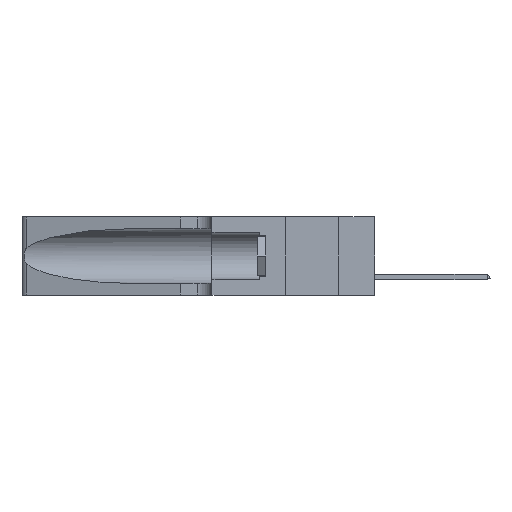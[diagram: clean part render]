
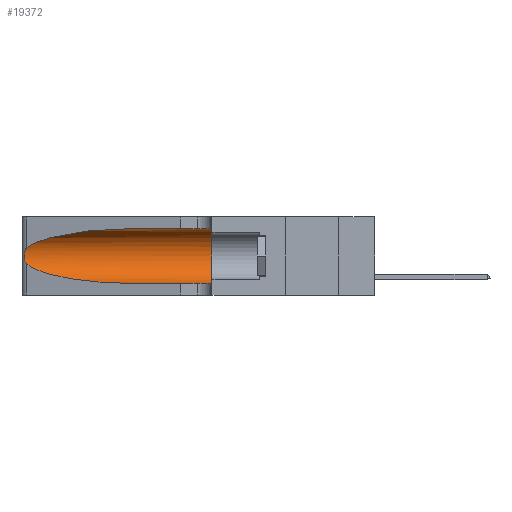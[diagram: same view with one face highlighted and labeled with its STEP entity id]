
A CAD part, left-side view. The second image highlights one B-rep face of the part: STEP entity #19372.
In plain terms, the highlighted cylindrical face has radius 3.308 mm (diameter 6.617 mm), a partial arc.
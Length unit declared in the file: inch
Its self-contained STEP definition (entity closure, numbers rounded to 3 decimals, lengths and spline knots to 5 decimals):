
#182 = DIRECTION ( 'NONE',  ( 0., -1., 0. ) ) ;
#310 = CARTESIAN_POINT ( 'NONE',  ( 0.18966, 0.96281, 0.31525 ) ) ;
#332 = DIRECTION ( 'NONE',  ( 0., -1., 0. ) ) ;
#604 = ORIENTED_EDGE ( 'NONE', *, *, #14429, .T. ) ;
#1430 = CIRCLE ( 'NONE', #5214, 0.13025 ) ;
#1632 = FACE_OUTER_BOUND ( 'NONE', #19201, .T. ) ;
#1670 = CARTESIAN_POINT ( 'NONE',  ( 0.1305, 0.72297, 0.05475 ) ) ;
#1849 = CARTESIAN_POINT ( 'NONE',  ( 0.1305, 1.61858, 0.05475 ) ) ;
#1985 = CARTESIAN_POINT ( 'NONE',  ( 0.1305, 0.35, 0.05475 ) ) ;
#2293 = CARTESIAN_POINT ( 'NONE',  ( 0.25854, 1.2359, 0.20912 ) ) ;
#2386 = CARTESIAN_POINT ( 'NONE',  ( 0.25639, 1.23186, 0.15144 ) ) ;
#2620 = CARTESIAN_POINT ( 'NONE',  ( 0.1305, 0.72297, 0.31525 ) ) ;
#3066 = CARTESIAN_POINT ( 'NONE',  ( 0.2373, 1.15595, 0.08982 ) ) ;
#3761 = EDGE_CURVE ( 'NONE', #15529, #11545, #9723, .T. ) ;
#4092 = ORIENTED_EDGE ( 'NONE', *, *, #24212, .T. ) ;
#4345 = CARTESIAN_POINT ( 'NONE',  ( 0.26075, 1.23896, 0.19203 ) ) ;
#4427 = CARTESIAN_POINT ( 'NONE',  ( 0.26075, 1.23896, 0.178 ) ) ;
#4687 = CARTESIAN_POINT ( 'NONE',  ( 0.26018, 1.23835, 0.19895 ) ) ;
#5214 = AXIS2_PLACEMENT_3D ( 'NONE', #21420, #5239, #23295 ) ;
#5239 = DIRECTION ( 'NONE',  ( 0., 1., 0. ) ) ;
#5252 = EDGE_CURVE ( 'NONE', #17333, #8176, #8739, .T. ) ;
#5857 = CARTESIAN_POINT ( 'NONE',  ( 0.1305, 1.61858, 0.31525 ) ) ;
#6425 = LINE ( 'NONE', #1849, #22662 ) ;
#6558 = ORIENTED_EDGE ( 'NONE', *, *, #5252, .F. ) ;
#6593 = CARTESIAN_POINT ( 'NONE',  ( 0.25487, 1.22718, 0.22369 ) ) ;
#6940 = EDGE_CURVE ( 'NONE', #8176, #10241, #1430, .T. ) ;
#8176 = VERTEX_POINT ( 'NONE', #21376 ) ;
#8487 = CARTESIAN_POINT ( 'NONE',  ( 0.25487, 1.22718, 0.14631 ) ) ;
#8548 = CARTESIAN_POINT ( 'NONE',  ( 0.2373, 1.15595, 0.28018 ) ) ;
#8578 = CARTESIAN_POINT ( 'NONE',  ( 0.25787, 1.23484, 0.2124 ) ) ;
#8739 = LINE ( 'NONE', #5857, #22819 ) ;
#8995 = CARTESIAN_POINT ( 'NONE',  ( 0.25487, 1.22718, 0.14631 ) ) ;
#9239 = VERTEX_POINT ( 'NONE', #20518 ) ;
#9723 =( BOUNDED_CURVE ( )  B_SPLINE_CURVE ( 3, ( #8995, #3066, #19226, #18870 ),
 .UNSPECIFIED., .F., .T. ) 
 B_SPLINE_CURVE_WITH_KNOTS ( ( 4, 4 ),
 ( 3.44316, 4.71239 ),
 .UNSPECIFIED. ) 
 CURVE ( )  GEOMETRIC_REPRESENTATION_ITEM ( )  RATIONAL_B_SPLINE_CURVE ( ( 1., 0.87, 0.87, 1. ) ) 
 REPRESENTATION_ITEM ( '' )  );
#10241 = VERTEX_POINT ( 'NONE', #1985 ) ;
#10252 = DIRECTION ( 'NONE',  ( 0., 0., -1. ) ) ;
#10747 = CARTESIAN_POINT ( 'NONE',  ( 0.1305, 0.72297, 0.31525 ) ) ;
#11545 = VERTEX_POINT ( 'NONE', #1670 ) ;
#11573 = ORIENTED_EDGE ( 'NONE', *, *, #22761, .T. ) ;
#11942 = DIRECTION ( 'NONE',  ( 0., -1., 0. ) ) ;
#14140 = CARTESIAN_POINT ( 'NONE',  ( 0.1305, 1.61858, 0.185 ) ) ;
#14429 = EDGE_CURVE ( 'NONE', #11545, #10241, #6425, .T. ) ;
#15529 = VERTEX_POINT ( 'NONE', #20856 ) ;
#16565 = CARTESIAN_POINT ( 'NONE',  ( 0.25487, 1.22718, 0.22369 ) ) ;
#16583 = B_SPLINE_CURVE_WITH_KNOTS ( 'NONE', 3,
 ( #6593, #20341, #24408, #8578, #2293, #4687, #4345, #4427, #20603, #22413, #18572, #2386, #18304, #8487 ),
 .UNSPECIFIED., .F., .F.,
 ( 4, 2, 2, 2, 2, 2, 4 ),
 ( 0., 0.00027, 0.00053, 0.00107, 0.0016, 0.00187, 0.00214 ),
 .UNSPECIFIED. ) ;
#17333 = VERTEX_POINT ( 'NONE', #10747 ) ;
#18304 = CARTESIAN_POINT ( 'NONE',  ( 0.25555, 1.22993, 0.14849 ) ) ;
#18572 = CARTESIAN_POINT ( 'NONE',  ( 0.25789, 1.23486, 0.15765 ) ) ;
#18870 = CARTESIAN_POINT ( 'NONE',  ( 0.1305, 0.72297, 0.05475 ) ) ;
#19201 = EDGE_LOOP ( 'NONE', ( #11573, #4092, #20908, #604, #19895, #6558 ) ) ;
#19226 = CARTESIAN_POINT ( 'NONE',  ( 0.18966, 0.96281, 0.05475 ) ) ;
#19372 = ADVANCED_FACE ( 'NONE', ( #1632 ), #19486, .F. ) ;
#19486 = CYLINDRICAL_SURFACE ( 'NONE', #20766, 0.13025 ) ;
#19895 = ORIENTED_EDGE ( 'NONE', *, *, #6940, .F. ) ;
#20341 = CARTESIAN_POINT ( 'NONE',  ( 0.25555, 1.22994, 0.2215 ) ) ;
#20518 = CARTESIAN_POINT ( 'NONE',  ( 0.25487, 1.22718, 0.22369 ) ) ;
#20603 = CARTESIAN_POINT ( 'NONE',  ( 0.26017, 1.23833, 0.17102 ) ) ;
#20766 = AXIS2_PLACEMENT_3D ( 'NONE', #14140, #332, #10252 ) ;
#20856 = CARTESIAN_POINT ( 'NONE',  ( 0.25487, 1.22718, 0.14631 ) ) ;
#20908 = ORIENTED_EDGE ( 'NONE', *, *, #3761, .T. ) ;
#21376 = CARTESIAN_POINT ( 'NONE',  ( 0.1305, 0.35, 0.31525 ) ) ;
#21420 = CARTESIAN_POINT ( 'NONE',  ( 0.1305, 0.35, 0.185 ) ) ;
#21766 =( BOUNDED_CURVE ( )  B_SPLINE_CURVE ( 3, ( #2620, #310, #8548, #16565 ),
 .UNSPECIFIED., .F., .F. ) 
 B_SPLINE_CURVE_WITH_KNOTS ( ( 4, 4 ),
 ( 1.5708, 2.84003 ),
 .UNSPECIFIED. ) 
 CURVE ( )  GEOMETRIC_REPRESENTATION_ITEM ( )  RATIONAL_B_SPLINE_CURVE ( ( 1., 0.87, 0.87, 1. ) ) 
 REPRESENTATION_ITEM ( '' )  );
#22413 = CARTESIAN_POINT ( 'NONE',  ( 0.25856, 1.23593, 0.16098 ) ) ;
#22662 = VECTOR ( 'NONE', #182, 39.37008 ) ;
#22761 = EDGE_CURVE ( 'NONE', #17333, #9239, #21766, .T. ) ;
#22819 = VECTOR ( 'NONE', #11942, 39.37008 ) ;
#23295 = DIRECTION ( 'NONE',  ( 0., 0., 1. ) ) ;
#24212 = EDGE_CURVE ( 'NONE', #9239, #15529, #16583, .T. ) ;
#24408 = CARTESIAN_POINT ( 'NONE',  ( 0.25639, 1.23184, 0.21858 ) ) ;
